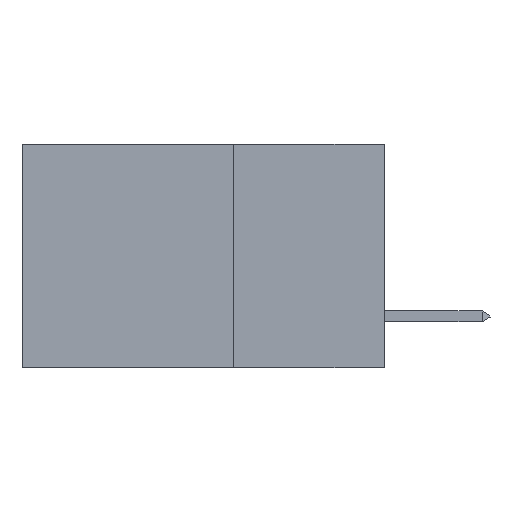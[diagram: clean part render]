
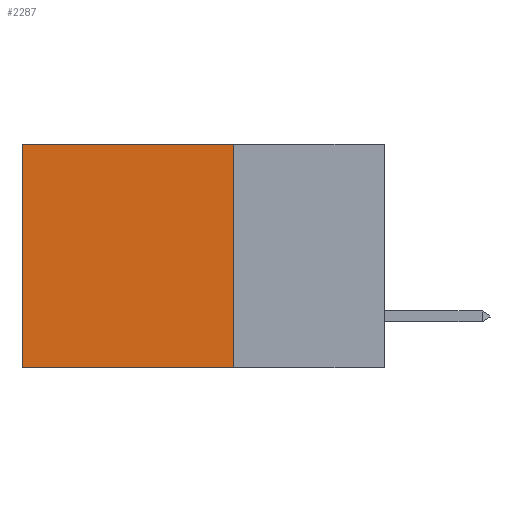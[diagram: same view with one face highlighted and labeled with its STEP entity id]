
A CAD part, left-side view. The second image highlights one B-rep face of the part: STEP entity #2287.
In plain terms, the highlighted planar face has unit normal (-1, 0, 0).
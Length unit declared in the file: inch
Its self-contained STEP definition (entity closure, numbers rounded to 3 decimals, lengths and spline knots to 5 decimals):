
#489 = DIRECTION ( 'NONE',  ( 0., 1., 0. ) ) ;
#1304 = FACE_OUTER_BOUND ( 'NONE', #10770, .T. ) ;
#1531 = CARTESIAN_POINT ( 'NONE',  ( 0.2875, 0.25, 0. ) ) ;
#1567 = DIRECTION ( 'NONE',  ( 0., 1., 0. ) ) ;
#2287 = ADVANCED_FACE ( 'NONE', ( #1304 ), #18067, .F. ) ;
#2365 = LINE ( 'NONE', #13341, #15280 ) ;
#2544 = VECTOR ( 'NONE', #489, 39.37008 ) ;
#3060 = VERTEX_POINT ( 'NONE', #12318 ) ;
#3236 = VERTEX_POINT ( 'NONE', #1531 ) ;
#4216 = ORIENTED_EDGE ( 'NONE', *, *, #11242, .T. ) ;
#5303 = VERTEX_POINT ( 'NONE', #9047 ) ;
#5443 = CARTESIAN_POINT ( 'NONE',  ( 0.2875, 0.6, 0. ) ) ;
#5528 = ORIENTED_EDGE ( 'NONE', *, *, #21477, .F. ) ;
#6317 = CARTESIAN_POINT ( 'NONE',  ( 0.2875, 0.25, 0. ) ) ;
#6362 = CARTESIAN_POINT ( 'NONE',  ( 0.2875, 0.25, 0. ) ) ;
#6998 = AXIS2_PLACEMENT_3D ( 'NONE', #6317, #11449, #11167 ) ;
#7223 = CARTESIAN_POINT ( 'NONE',  ( 0.2875, 0.25, 0. ) ) ;
#8033 = DIRECTION ( 'NONE',  ( 0., 0., -1. ) ) ;
#9047 = CARTESIAN_POINT ( 'NONE',  ( 0.2875, 0.6, -0.37 ) ) ;
#9423 = VECTOR ( 'NONE', #13745, 39.37008 ) ;
#9599 = ORIENTED_EDGE ( 'NONE', *, *, #15631, .T. ) ;
#10190 = LINE ( 'NONE', #7223, #2544 ) ;
#10770 = EDGE_LOOP ( 'NONE', ( #4216, #15107, #5528, #9599 ) ) ;
#11120 = EDGE_CURVE ( 'NONE', #3060, #5303, #2365, .T. ) ;
#11167 = DIRECTION ( 'NONE',  ( 0., 0., -1. ) ) ;
#11242 = EDGE_CURVE ( 'NONE', #21722, #5303, #20674, .T. ) ;
#11449 = DIRECTION ( 'NONE',  ( 1., 0., 0. ) ) ;
#12318 = CARTESIAN_POINT ( 'NONE',  ( 0.2875, 0.25, -0.37 ) ) ;
#12678 = CARTESIAN_POINT ( 'NONE',  ( 0.2875, 0.6, 0. ) ) ;
#12784 = VECTOR ( 'NONE', #8033, 39.37008 ) ;
#13341 = CARTESIAN_POINT ( 'NONE',  ( 0.2875, 0.25, -0.37 ) ) ;
#13745 = DIRECTION ( 'NONE',  ( 0., 0., -1. ) ) ;
#15107 = ORIENTED_EDGE ( 'NONE', *, *, #11120, .F. ) ;
#15280 = VECTOR ( 'NONE', #1567, 39.37008 ) ;
#15631 = EDGE_CURVE ( 'NONE', #3236, #21722, #10190, .T. ) ;
#18067 = PLANE ( 'NONE',  #6998 ) ;
#20674 = LINE ( 'NONE', #12678, #9423 ) ;
#21477 = EDGE_CURVE ( 'NONE', #3236, #3060, #21697, .T. ) ;
#21697 = LINE ( 'NONE', #6362, #12784 ) ;
#21722 = VERTEX_POINT ( 'NONE', #5443 ) ;
